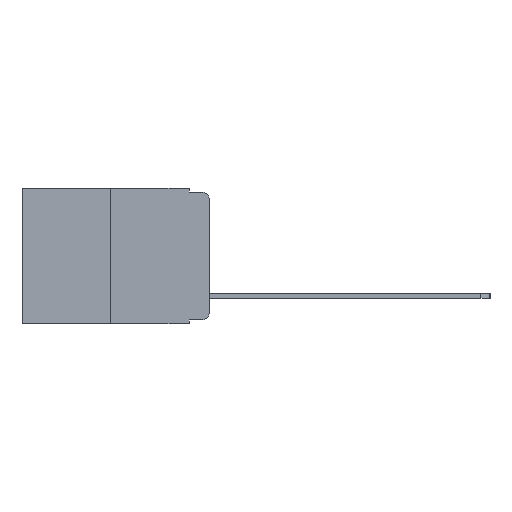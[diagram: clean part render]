
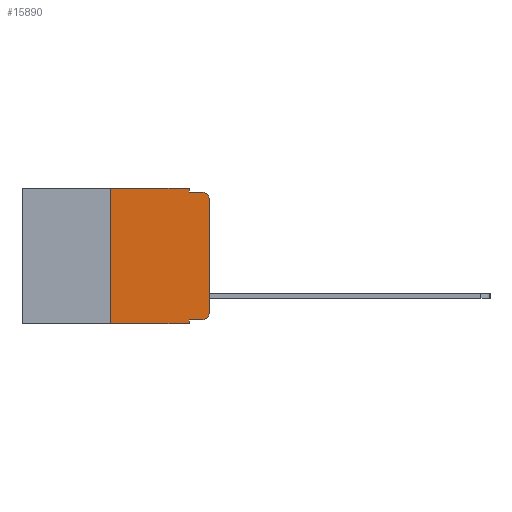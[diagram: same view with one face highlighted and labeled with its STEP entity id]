
A CAD part, left-side view. The second image highlights one B-rep face of the part: STEP entity #15890.
In plain terms, the highlighted planar face has unit normal (-1, 0, 0).
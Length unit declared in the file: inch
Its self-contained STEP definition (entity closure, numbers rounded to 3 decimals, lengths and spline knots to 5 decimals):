
#752 = CARTESIAN_POINT ( 'NONE',  ( 0., 0.02, -0.01 ) ) ;
#1082 = LINE ( 'NONE', #5100, #14494 ) ;
#1291 = ORIENTED_EDGE ( 'NONE', *, *, #15385, .T. ) ;
#1507 = ORIENTED_EDGE ( 'NONE', *, *, #14260, .T. ) ;
#1611 = ORIENTED_EDGE ( 'NONE', *, *, #11998, .F. ) ;
#1775 = ORIENTED_EDGE ( 'NONE', *, *, #10813, .F. ) ;
#1798 = ORIENTED_EDGE ( 'NONE', *, *, #18137, .F. ) ;
#1911 = ORIENTED_EDGE ( 'NONE', *, *, #9667, .F. ) ;
#1976 = ORIENTED_EDGE ( 'NONE', *, *, #12284, .T. ) ;
#2207 = CARTESIAN_POINT ( 'NONE',  ( 0., 0.473, 0. ) ) ;
#2245 = ORIENTED_EDGE ( 'NONE', *, *, #8530, .F. ) ;
#2442 = ORIENTED_EDGE ( 'NONE', *, *, #7358, .T. ) ;
#2619 = ORIENTED_EDGE ( 'NONE', *, *, #6187, .T. ) ;
#2687 = CARTESIAN_POINT ( 'NONE',  ( 0., 0.051, -0.01 ) ) ;
#3737 = LINE ( 'NONE', #8551, #11340 ) ;
#4268 = VECTOR ( 'NONE', #20013, 39.37008 ) ;
#4283 = CARTESIAN_POINT ( 'NONE',  ( 0., 0.02, -0.03 ) ) ;
#4365 = CARTESIAN_POINT ( 'NONE',  ( 0., 0., -0.313 ) ) ;
#4522 = DIRECTION ( 'NONE',  ( -1., 0., 0. ) ) ;
#4839 = VERTEX_POINT ( 'NONE', #12727 ) ;
#5100 = CARTESIAN_POINT ( 'NONE',  ( 0., 0.051, -0.01 ) ) ;
#6039 = DIRECTION ( 'NONE',  ( 0., 0., -1. ) ) ;
#6187 = EDGE_CURVE ( 'NONE', #9391, #7240, #12925, .T. ) ;
#6895 = CARTESIAN_POINT ( 'NONE',  ( 0., 0.25, -0.343 ) ) ;
#6957 = VECTOR ( 'NONE', #10076, 39.37008 ) ;
#7110 = CARTESIAN_POINT ( 'NONE',  ( 0., 0.051, -0.343 ) ) ;
#7240 = VERTEX_POINT ( 'NONE', #4365 ) ;
#7358 = EDGE_CURVE ( 'NONE', #19109, #9391, #8358, .T. ) ;
#7458 = DIRECTION ( 'NONE',  ( 1., 0., 0. ) ) ;
#7695 = DIRECTION ( 'NONE',  ( 0., 0., 1. ) ) ;
#7870 = DIRECTION ( 'NONE',  ( 0., -1., 0. ) ) ;
#8044 = VECTOR ( 'NONE', #7695, 39.37008 ) ;
#8244 = CARTESIAN_POINT ( 'NONE',  ( 0., 0.051, -0.333 ) ) ;
#8358 = LINE ( 'NONE', #8244, #4268 ) ;
#8530 = EDGE_CURVE ( 'NONE', #19109, #18597, #16010, .T. ) ;
#8551 = CARTESIAN_POINT ( 'NONE',  ( 0., 0.051, 0. ) ) ;
#8584 = LINE ( 'NONE', #14711, #21412 ) ;
#8963 = LINE ( 'NONE', #2207, #17412 ) ;
#9391 = VERTEX_POINT ( 'NONE', #20731 ) ;
#9667 = EDGE_CURVE ( 'NONE', #19187, #20626, #17402, .T. ) ;
#9821 = CARTESIAN_POINT ( 'NONE',  ( 0., 0.25, 0. ) ) ;
#10076 = DIRECTION ( 'NONE',  ( 0., 0., -1. ) ) ;
#10428 = FACE_OUTER_BOUND ( 'NONE', #19223, .T. ) ;
#10813 = EDGE_CURVE ( 'NONE', #4839, #18951, #3737, .T. ) ;
#11340 = VECTOR ( 'NONE', #20308, 39.37008 ) ;
#11394 = CARTESIAN_POINT ( 'NONE',  ( 0., 0., -0.03 ) ) ;
#11824 = CARTESIAN_POINT ( 'NONE',  ( 0., 0.051, 0. ) ) ;
#11998 = EDGE_CURVE ( 'NONE', #18951, #12333, #1082, .T. ) ;
#12284 = EDGE_CURVE ( 'NONE', #19187, #18597, #8584, .T. ) ;
#12333 = VERTEX_POINT ( 'NONE', #752 ) ;
#12727 = CARTESIAN_POINT ( 'NONE',  ( 0., 0.051, 0. ) ) ;
#12852 = AXIS2_PLACEMENT_3D ( 'NONE', #14841, #4522, #16485 ) ;
#12925 = CIRCLE ( 'NONE', #12852, 0.02 ) ;
#14260 = EDGE_CURVE ( 'NONE', #18801, #12333, #17231, .T. ) ;
#14494 = VECTOR ( 'NONE', #17015, 39.37008 ) ;
#14711 = CARTESIAN_POINT ( 'NONE',  ( 0., 0.473, -0.343 ) ) ;
#14841 = CARTESIAN_POINT ( 'NONE',  ( 0., 0.02, -0.313 ) ) ;
#15385 = EDGE_CURVE ( 'NONE', #7240, #18801, #17577, .T. ) ;
#15890 = ADVANCED_FACE ( 'NONE', ( #10428 ), #15951, .F. ) ;
#15951 = PLANE ( 'NONE',  #19946 ) ;
#16010 = LINE ( 'NONE', #11824, #6957 ) ;
#16260 = DIRECTION ( 'NONE',  ( -1., 0., 0. ) ) ;
#16485 = DIRECTION ( 'NONE',  ( 0., 0., -1. ) ) ;
#17015 = DIRECTION ( 'NONE',  ( 0., -1., 0. ) ) ;
#17231 = CIRCLE ( 'NONE', #21267, 0.02 ) ;
#17402 = LINE ( 'NONE', #9821, #21765 ) ;
#17412 = VECTOR ( 'NONE', #20932, 39.37008 ) ;
#17577 = LINE ( 'NONE', #21126, #8044 ) ;
#17596 = CARTESIAN_POINT ( 'NONE',  ( 0., 0.473, 0. ) ) ;
#18137 = EDGE_CURVE ( 'NONE', #20626, #4839, #8963, .T. ) ;
#18597 = VERTEX_POINT ( 'NONE', #7110 ) ;
#18801 = VERTEX_POINT ( 'NONE', #11394 ) ;
#18951 = VERTEX_POINT ( 'NONE', #2687 ) ;
#19043 = CARTESIAN_POINT ( 'NONE',  ( 0., 0.25, 0. ) ) ;
#19109 = VERTEX_POINT ( 'NONE', #21867 ) ;
#19187 = VERTEX_POINT ( 'NONE', #6895 ) ;
#19223 = EDGE_LOOP ( 'NONE', ( #1291, #1507, #1611, #1775, #1798, #1911, #1976, #2245, #2442, #2619 ) ) ;
#19246 = DIRECTION ( 'NONE',  ( 0., 0., -1. ) ) ;
#19859 = DIRECTION ( 'NONE',  ( 0., 0., 1. ) ) ;
#19946 = AXIS2_PLACEMENT_3D ( 'NONE', #17596, #7458, #19246 ) ;
#20013 = DIRECTION ( 'NONE',  ( 0., -1., 0. ) ) ;
#20308 = DIRECTION ( 'NONE',  ( 0., 0., -1. ) ) ;
#20626 = VERTEX_POINT ( 'NONE', #19043 ) ;
#20731 = CARTESIAN_POINT ( 'NONE',  ( 0., 0.02, -0.333 ) ) ;
#20932 = DIRECTION ( 'NONE',  ( 0., -1., 0. ) ) ;
#21126 = CARTESIAN_POINT ( 'NONE',  ( 0., 0., 0. ) ) ;
#21267 = AXIS2_PLACEMENT_3D ( 'NONE', #4283, #16260, #6039 ) ;
#21412 = VECTOR ( 'NONE', #7870, 39.37008 ) ;
#21765 = VECTOR ( 'NONE', #19859, 39.37008 ) ;
#21867 = CARTESIAN_POINT ( 'NONE',  ( 0., 0.051, -0.333 ) ) ;
